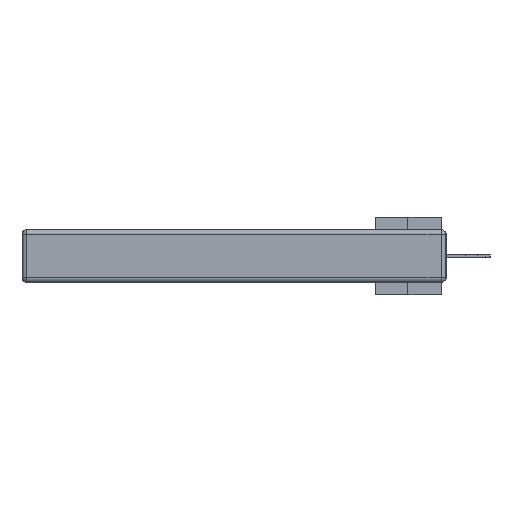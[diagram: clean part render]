
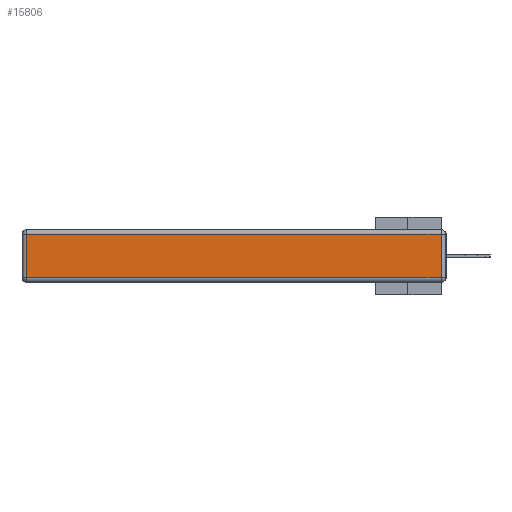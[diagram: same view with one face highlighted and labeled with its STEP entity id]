
A CAD part, left-side view. The second image highlights one B-rep face of the part: STEP entity #15806.
In plain terms, the highlighted planar face has unit normal (-1, 0, 0).
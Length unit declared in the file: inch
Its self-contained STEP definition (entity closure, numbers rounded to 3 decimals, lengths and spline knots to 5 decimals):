
#1321 = LINE ( 'NONE', #22964, #26831 ) ;
#1419 = CARTESIAN_POINT ( 'NONE',  ( 0., 0., -0.313 ) ) ;
#1487 = CARTESIAN_POINT ( 'NONE',  ( 0., 0., -0.343 ) ) ;
#2055 = DIRECTION ( 'NONE',  ( 0., 0., -1. ) ) ;
#3602 = LINE ( 'NONE', #1419, #35055 ) ;
#5581 = DIRECTION ( 'NONE',  ( 0., 0., 1. ) ) ;
#8842 = ORIENTED_EDGE ( 'NONE', *, *, #16922, .T. ) ;
#9118 = EDGE_CURVE ( 'NONE', #14707, #18382, #17770, .T. ) ;
#9723 = DIRECTION ( 'NONE',  ( 0., -1., 0. ) ) ;
#12837 = EDGE_CURVE ( 'NONE', #31205, #14707, #17468, .T. ) ;
#14707 = VERTEX_POINT ( 'NONE', #17449 ) ;
#14837 = DIRECTION ( 'NONE',  ( 0., 0., 1. ) ) ;
#15213 = CARTESIAN_POINT ( 'NONE',  ( 0., 2.72, -0.343 ) ) ;
#15478 = CARTESIAN_POINT ( 'NONE',  ( 0., 2.75, -0.03 ) ) ;
#15806 = ADVANCED_FACE ( 'NONE', ( #20618 ), #26200, .T. ) ;
#16922 = EDGE_CURVE ( 'NONE', #19529, #31205, #1321, .T. ) ;
#17449 = CARTESIAN_POINT ( 'NONE',  ( 0., 2.72, -0.03 ) ) ;
#17468 = LINE ( 'NONE', #15478, #27705 ) ;
#17770 = LINE ( 'NONE', #15213, #33740 ) ;
#18382 = VERTEX_POINT ( 'NONE', #29481 ) ;
#19119 = EDGE_LOOP ( 'NONE', ( #22405, #8842, #26457, #22677 ) ) ;
#19529 = VERTEX_POINT ( 'NONE', #28949 ) ;
#20618 = FACE_OUTER_BOUND ( 'NONE', #19119, .T. ) ;
#22405 = ORIENTED_EDGE ( 'NONE', *, *, #22920, .T. ) ;
#22677 = ORIENTED_EDGE ( 'NONE', *, *, #9118, .T. ) ;
#22920 = EDGE_CURVE ( 'NONE', #18382, #19529, #3602, .T. ) ;
#22964 = CARTESIAN_POINT ( 'NONE',  ( 0., 0.03, -0.343 ) ) ;
#25435 = CARTESIAN_POINT ( 'NONE',  ( 0., 0.03, -0.03 ) ) ;
#26200 = PLANE ( 'NONE',  #35549 ) ;
#26457 = ORIENTED_EDGE ( 'NONE', *, *, #12837, .T. ) ;
#26831 = VECTOR ( 'NONE', #14837, 39.37008 ) ;
#27236 = DIRECTION ( 'NONE',  ( -1., 0., 0. ) ) ;
#27705 = VECTOR ( 'NONE', #31555, 39.37008 ) ;
#28949 = CARTESIAN_POINT ( 'NONE',  ( 0., 0.03, -0.313 ) ) ;
#29481 = CARTESIAN_POINT ( 'NONE',  ( 0., 2.72, -0.313 ) ) ;
#31205 = VERTEX_POINT ( 'NONE', #25435 ) ;
#31555 = DIRECTION ( 'NONE',  ( 0., 1., 0. ) ) ;
#33740 = VECTOR ( 'NONE', #2055, 39.37008 ) ;
#35055 = VECTOR ( 'NONE', #9723, 39.37008 ) ;
#35549 = AXIS2_PLACEMENT_3D ( 'NONE', #1487, #27236, #5581 ) ;
